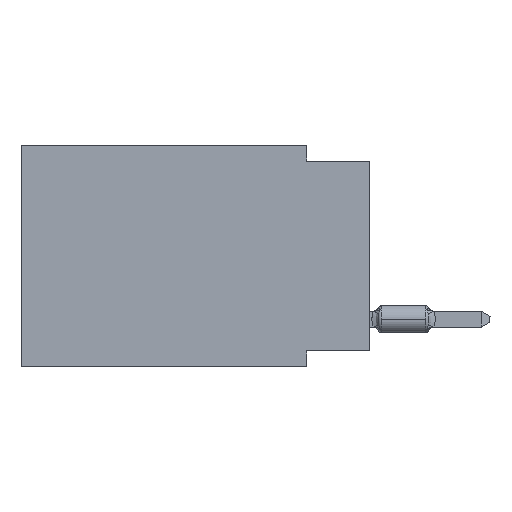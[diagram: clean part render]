
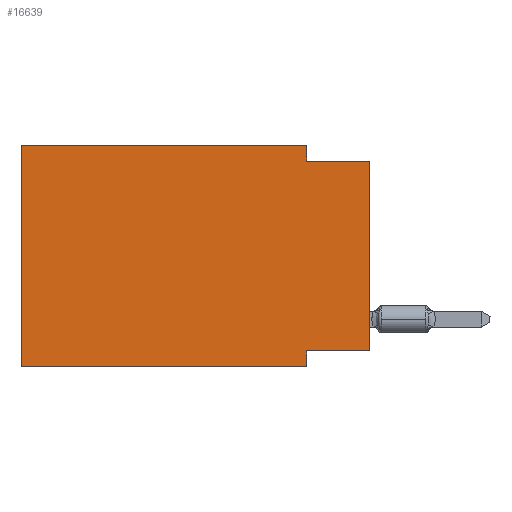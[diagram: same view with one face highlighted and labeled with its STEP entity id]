
A CAD part, left-side view. The second image highlights one B-rep face of the part: STEP entity #16639.
In plain terms, the highlighted planar face has unit normal (-1, 0, 0).
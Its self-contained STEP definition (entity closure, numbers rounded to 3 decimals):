
#677 = VECTOR ( 'NONE', #3108, 1000. ) ;
#3108 = DIRECTION ( 'NONE',  ( 0., 0., 1. ) ) ;
#3214 = CARTESIAN_POINT ( 'NONE',  ( 0., 13.97, 0. ) ) ;
#4737 = CARTESIAN_POINT ( 'NONE',  ( 0., 0., -0.635 ) ) ;
#5133 = EDGE_CURVE ( 'NONE', #97161, #22715, #70548, .T. ) ;
#5408 = DIRECTION ( 'NONE',  ( 0., 0., 1. ) ) ;
#6781 = EDGE_CURVE ( 'NONE', #97161, #11285, #44626, .T. ) ;
#8231 = VECTOR ( 'NONE', #37457, 1000. ) ;
#8883 = LINE ( 'NONE', #33948, #65901 ) ;
#9223 = ORIENTED_EDGE ( 'NONE', *, *, #14099, .F. ) ;
#10766 = EDGE_CURVE ( 'NONE', #36488, #89910, #28964, .T. ) ;
#11285 = VERTEX_POINT ( 'NONE', #106827 ) ;
#11727 = DIRECTION ( 'NONE',  ( 0., -1., 0. ) ) ;
#12014 = CARTESIAN_POINT ( 'NONE',  ( 0., 2.54, -8.89 ) ) ;
#12698 = ORIENTED_EDGE ( 'NONE', *, *, #70034, .F. ) ;
#13292 = VERTEX_POINT ( 'NONE', #12014 ) ;
#13625 = VECTOR ( 'NONE', #95155, 1000. ) ;
#14099 = EDGE_CURVE ( 'NONE', #80866, #22715, #8883, .T. ) ;
#16639 = ADVANCED_FACE ( 'NONE', ( #29244 ), #54342, .F. ) ;
#17269 = CARTESIAN_POINT ( 'NONE',  ( 0., 13.97, -8.89 ) ) ;
#22715 = VERTEX_POINT ( 'NONE', #4737 ) ;
#24748 = CARTESIAN_POINT ( 'NONE',  ( 0., 2.54, -0.635 ) ) ;
#24994 = CARTESIAN_POINT ( 'NONE',  ( 0., 2.54, 0. ) ) ;
#25067 = LINE ( 'NONE', #17269, #90095 ) ;
#25584 = DIRECTION ( 'NONE',  ( 0., -1., 0. ) ) ;
#25878 = CARTESIAN_POINT ( 'NONE',  ( 0., 13.97, -8.89 ) ) ;
#27161 = AXIS2_PLACEMENT_3D ( 'NONE', #28696, #89386, #98295 ) ;
#28696 = CARTESIAN_POINT ( 'NONE',  ( 0., 13.97, 0. ) ) ;
#28774 = ORIENTED_EDGE ( 'NONE', *, *, #30524, .F. ) ;
#28964 = LINE ( 'NONE', #72436, #88463 ) ;
#29244 = FACE_OUTER_BOUND ( 'NONE', #66452, .T. ) ;
#30524 = EDGE_CURVE ( 'NONE', #89910, #80866, #61172, .T. ) ;
#30674 = ORIENTED_EDGE ( 'NONE', *, *, #83996, .T. ) ;
#33948 = CARTESIAN_POINT ( 'NONE',  ( 0., 0., -0.635 ) ) ;
#36488 = VERTEX_POINT ( 'NONE', #86942 ) ;
#37457 = DIRECTION ( 'NONE',  ( 0., 0., -1. ) ) ;
#38119 = VECTOR ( 'NONE', #101487, 1000. ) ;
#44626 = LINE ( 'NONE', #67506, #38119 ) ;
#45205 = ORIENTED_EDGE ( 'NONE', *, *, #6781, .F. ) ;
#48062 = ORIENTED_EDGE ( 'NONE', *, *, #10766, .F. ) ;
#48571 = EDGE_CURVE ( 'NONE', #11285, #13292, #105988, .T. ) ;
#54342 = PLANE ( 'NONE',  #27161 ) ;
#54808 = CARTESIAN_POINT ( 'NONE',  ( 0., 2.54, 0. ) ) ;
#59053 = DIRECTION ( 'NONE',  ( 0., -1., 0. ) ) ;
#61172 = LINE ( 'NONE', #24994, #13625 ) ;
#64342 = VECTOR ( 'NONE', #5408, 1000. ) ;
#65901 = VECTOR ( 'NONE', #25584, 1000. ) ;
#66452 = EDGE_LOOP ( 'NONE', ( #97239, #9223, #28774, #48062, #12698, #30674, #78807, #45205 ) ) ;
#67506 = CARTESIAN_POINT ( 'NONE',  ( 0., 0., -8.255 ) ) ;
#70034 = EDGE_CURVE ( 'NONE', #88132, #36488, #71200, .T. ) ;
#70548 = LINE ( 'NONE', #96697, #677 ) ;
#71200 = LINE ( 'NONE', #3214, #64342 ) ;
#72436 = CARTESIAN_POINT ( 'NONE',  ( 0., 13.97, 0. ) ) ;
#78807 = ORIENTED_EDGE ( 'NONE', *, *, #48571, .F. ) ;
#80866 = VERTEX_POINT ( 'NONE', #24748 ) ;
#83996 = EDGE_CURVE ( 'NONE', #88132, #13292, #25067, .T. ) ;
#86942 = CARTESIAN_POINT ( 'NONE',  ( 0., 13.97, 0. ) ) ;
#88132 = VERTEX_POINT ( 'NONE', #25878 ) ;
#88463 = VECTOR ( 'NONE', #11727, 1000. ) ;
#89386 = DIRECTION ( 'NONE',  ( 1., 0., 0. ) ) ;
#89910 = VERTEX_POINT ( 'NONE', #54808 ) ;
#90095 = VECTOR ( 'NONE', #59053, 1000. ) ;
#95155 = DIRECTION ( 'NONE',  ( 0., 0., -1. ) ) ;
#96697 = CARTESIAN_POINT ( 'NONE',  ( 0., 0., 0. ) ) ;
#97161 = VERTEX_POINT ( 'NONE', #103323 ) ;
#97239 = ORIENTED_EDGE ( 'NONE', *, *, #5133, .T. ) ;
#98152 = CARTESIAN_POINT ( 'NONE',  ( 0., 2.54, -8.89 ) ) ;
#98295 = DIRECTION ( 'NONE',  ( 0., 0., -1. ) ) ;
#101487 = DIRECTION ( 'NONE',  ( 0., 1., 0. ) ) ;
#103323 = CARTESIAN_POINT ( 'NONE',  ( 0., 0., -8.255 ) ) ;
#105988 = LINE ( 'NONE', #98152, #8231 ) ;
#106827 = CARTESIAN_POINT ( 'NONE',  ( 0., 2.54, -8.255 ) ) ;
